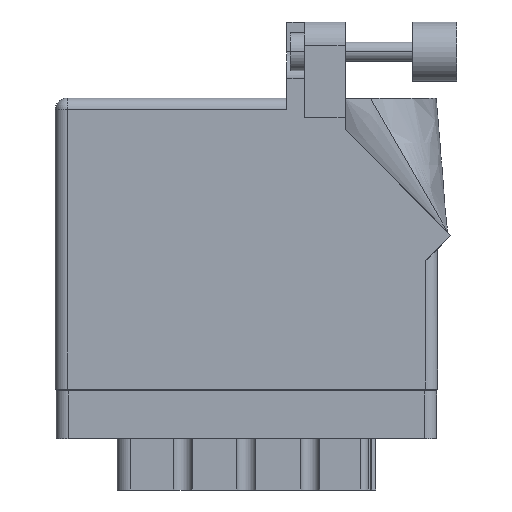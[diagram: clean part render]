
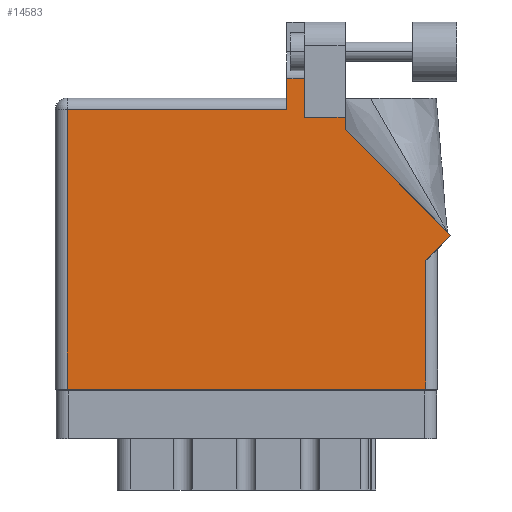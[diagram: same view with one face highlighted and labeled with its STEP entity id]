
A CAD part, front view. The second image highlights one B-rep face of the part: STEP entity #14583.
In plain terms, the highlighted face is planar.
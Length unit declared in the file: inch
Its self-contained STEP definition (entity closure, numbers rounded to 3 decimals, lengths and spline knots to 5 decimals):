
#189 = VECTOR ( 'NONE', #32463, 39.37008 ) ;
#295 = LINE ( 'NONE', #11838, #9352 ) ;
#335 = ORIENTED_EDGE ( 'NONE', *, *, #11655, .T. ) ;
#812 = EDGE_CURVE ( 'NONE', #23071, #14784, #12029, .T. ) ;
#1052 = CARTESIAN_POINT ( 'NONE',  ( 1.217, 1.6315, 0. ) ) ;
#1277 = LINE ( 'NONE', #18348, #10847 ) ;
#1561 = VERTEX_POINT ( 'NONE', #22769 ) ;
#2192 = ORIENTED_EDGE ( 'NONE', *, *, #19281, .T. ) ;
#2262 = DIRECTION ( 'NONE',  ( -1., 0., 0. ) ) ;
#3669 = VERTEX_POINT ( 'NONE', #15661 ) ;
#5682 = LINE ( 'NONE', #18835, #25536 ) ;
#6587 = VECTOR ( 'NONE', #35420, 39.37008 ) ;
#6657 = CARTESIAN_POINT ( 'NONE',  ( 1.217, 1.468, 0. ) ) ;
#7291 = VECTOR ( 'NONE', #30121, 39.37008 ) ;
#7436 = VERTEX_POINT ( 'NONE', #6657 ) ;
#7757 = ORIENTED_EDGE ( 'NONE', *, *, #812, .T. ) ;
#7960 = CARTESIAN_POINT ( 'NONE',  ( 0., 1.53, 0. ) ) ;
#8067 = EDGE_CURVE ( 'NONE', #14784, #21333, #19314, .T. ) ;
#8506 = ORIENTED_EDGE ( 'NONE', *, *, #19588, .T. ) ;
#8904 = CARTESIAN_POINT ( 'NONE',  ( 1.217, 1.53, 0. ) ) ;
#9063 = DIRECTION ( 'NONE',  ( -1., 0., 0. ) ) ;
#9198 = CARTESIAN_POINT ( 'NONE',  ( 1.948, 0.737, 0. ) ) ;
#9352 = VECTOR ( 'NONE', #12210, 39.37008 ) ;
#9710 = DIRECTION ( 'NONE',  ( 0., 1., 0. ) ) ;
#10847 = VECTOR ( 'NONE', #21570, 39.37008 ) ;
#10910 = VECTOR ( 'NONE', #29598, 39.37008 ) ;
#11655 = EDGE_CURVE ( 'NONE', #18809, #7436, #20675, .T. ) ;
#11723 = CARTESIAN_POINT ( 'NONE',  ( 1.948, 0.675, 0. ) ) ;
#11729 = LINE ( 'NONE', #17997, #10910 ) ;
#11802 = EDGE_CURVE ( 'NONE', #23263, #20177, #30158, .T. ) ;
#11838 = CARTESIAN_POINT ( 'NONE',  ( 0., 1.468, 0. ) ) ;
#12029 = LINE ( 'NONE', #9198, #6587 ) ;
#12123 = VECTOR ( 'NONE', #36993, 39.37008 ) ;
#12210 = DIRECTION ( 'NONE',  ( -1., 0., 0. ) ) ;
#12434 = LINE ( 'NONE', #15863, #7291 ) ;
#12984 = CARTESIAN_POINT ( 'NONE',  ( 1.524, 1.43, 0. ) ) ;
#14583 = ADVANCED_FACE ( 'NONE', ( #25804 ), #16499, .F. ) ;
#14784 = VERTEX_POINT ( 'NONE', #11723 ) ;
#15616 = CARTESIAN_POINT ( 'NONE',  ( 0.062, 1.468, 0. ) ) ;
#15661 = CARTESIAN_POINT ( 'NONE',  ( 0.062, 0., 0. ) ) ;
#15863 = CARTESIAN_POINT ( 'NONE',  ( 0., 0., 0. ) ) ;
#16499 = PLANE ( 'NONE',  #22297 ) ;
#16532 = VECTOR ( 'NONE', #32280, 39.37008 ) ;
#16586 = ORIENTED_EDGE ( 'NONE', *, *, #11802, .T. ) ;
#16866 = VERTEX_POINT ( 'NONE', #15616 ) ;
#17750 = CARTESIAN_POINT ( 'NONE',  ( 1.524, 1.36442, 0. ) ) ;
#17993 = ORIENTED_EDGE ( 'NONE', *, *, #31892, .T. ) ;
#17997 = CARTESIAN_POINT ( 'NONE',  ( 2.08071, 0.80771, 0. ) ) ;
#18255 = EDGE_CURVE ( 'NONE', #21333, #23263, #11729, .T. ) ;
#18276 = VECTOR ( 'NONE', #30344, 39.37008 ) ;
#18348 = CARTESIAN_POINT ( 'NONE',  ( 0.062, 0., 0. ) ) ;
#18629 = CARTESIAN_POINT ( 'NONE',  ( 1.311, 1.43, 0. ) ) ;
#18809 = VERTEX_POINT ( 'NONE', #1052 ) ;
#18835 = CARTESIAN_POINT ( 'NONE',  ( 1.64177, 1.6315, 0. ) ) ;
#18921 = CARTESIAN_POINT ( 'NONE',  ( 1.524, 1.43, 0. ) ) ;
#19281 = EDGE_CURVE ( 'NONE', #33092, #1561, #24152, .T. ) ;
#19314 = LINE ( 'NONE', #37356, #12123 ) ;
#19588 = EDGE_CURVE ( 'NONE', #20177, #33092, #25010, .T. ) ;
#19942 = CARTESIAN_POINT ( 'NONE',  ( 1.311, 1.43, 0. ) ) ;
#20177 = VERTEX_POINT ( 'NONE', #12984 ) ;
#20675 = LINE ( 'NONE', #8904, #16532 ) ;
#20943 = ORIENTED_EDGE ( 'NONE', *, *, #8067, .T. ) ;
#21229 = CARTESIAN_POINT ( 'NONE',  ( 2.08071, 0.80771, 0. ) ) ;
#21333 = VERTEX_POINT ( 'NONE', #21229 ) ;
#21570 = DIRECTION ( 'NONE',  ( 0., -1., 0. ) ) ;
#22297 = AXIS2_PLACEMENT_3D ( 'NONE', #7960, #37383, #2262 ) ;
#22331 = CARTESIAN_POINT ( 'NONE',  ( 1.948, 0., 0. ) ) ;
#22769 = CARTESIAN_POINT ( 'NONE',  ( 1.311, 1.6315, 0. ) ) ;
#23071 = VERTEX_POINT ( 'NONE', #22331 ) ;
#23263 = VERTEX_POINT ( 'NONE', #17750 ) ;
#23969 = ORIENTED_EDGE ( 'NONE', *, *, #27146, .T. ) ;
#24152 = LINE ( 'NONE', #18629, #32216 ) ;
#25010 = LINE ( 'NONE', #18921, #18276 ) ;
#25536 = VECTOR ( 'NONE', #9063, 39.37008 ) ;
#25804 = FACE_OUTER_BOUND ( 'NONE', #32457, .T. ) ;
#27146 = EDGE_CURVE ( 'NONE', #7436, #16866, #295, .T. ) ;
#28740 = ORIENTED_EDGE ( 'NONE', *, *, #18255, .T. ) ;
#29598 = DIRECTION ( 'NONE',  ( -0.707, 0.707, 0. ) ) ;
#29693 = ORIENTED_EDGE ( 'NONE', *, *, #34653, .T. ) ;
#30121 = DIRECTION ( 'NONE',  ( 1., 0., 0. ) ) ;
#30158 = LINE ( 'NONE', #35490, #189 ) ;
#30344 = DIRECTION ( 'NONE',  ( -1., 0., 0. ) ) ;
#31892 = EDGE_CURVE ( 'NONE', #1561, #18809, #5682, .T. ) ;
#31956 = EDGE_CURVE ( 'NONE', #16866, #3669, #1277, .T. ) ;
#32216 = VECTOR ( 'NONE', #9710, 39.37008 ) ;
#32280 = DIRECTION ( 'NONE',  ( 0., -1., 0. ) ) ;
#32457 = EDGE_LOOP ( 'NONE', ( #2192, #17993, #335, #23969, #35138, #29693, #7757, #20943, #28740, #16586, #8506 ) ) ;
#32463 = DIRECTION ( 'NONE',  ( 0., 1., 0. ) ) ;
#33092 = VERTEX_POINT ( 'NONE', #19942 ) ;
#34653 = EDGE_CURVE ( 'NONE', #3669, #23071, #12434, .T. ) ;
#35138 = ORIENTED_EDGE ( 'NONE', *, *, #31956, .T. ) ;
#35420 = DIRECTION ( 'NONE',  ( 0., 1., 0. ) ) ;
#35490 = CARTESIAN_POINT ( 'NONE',  ( 1.524, 1.36442, 0. ) ) ;
#36993 = DIRECTION ( 'NONE',  ( 0.707, 0.707, 0. ) ) ;
#37356 = CARTESIAN_POINT ( 'NONE',  ( 2.01, 0.737, 0. ) ) ;
#37383 = DIRECTION ( 'NONE',  ( 0., 0., -1. ) ) ;
